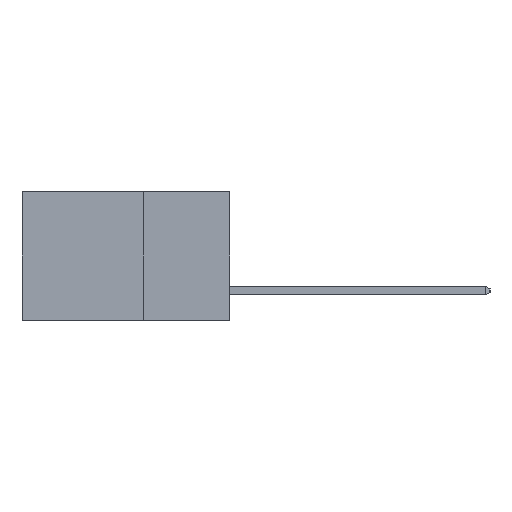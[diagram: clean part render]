
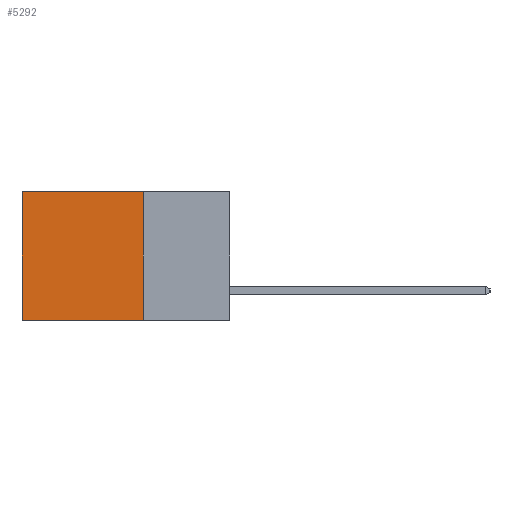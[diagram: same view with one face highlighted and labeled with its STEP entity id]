
A CAD part, left-side view. The second image highlights one B-rep face of the part: STEP entity #5292.
In plain terms, the highlighted planar face has unit normal (-1, 0, 0).
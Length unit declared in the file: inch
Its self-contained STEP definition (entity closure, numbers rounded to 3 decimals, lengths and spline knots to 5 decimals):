
#74 = VECTOR ( 'NONE', #10549, 39.37008 ) ;
#1083 = DIRECTION ( 'NONE',  ( 0., 0., -1. ) ) ;
#1556 = EDGE_CURVE ( 'NONE', #17391, #4035, #14110, .T. ) ;
#2933 = CARTESIAN_POINT ( 'NONE',  ( 0.298, 0.25, 0. ) ) ;
#3402 = VECTOR ( 'NONE', #12834, 39.37008 ) ;
#4035 = VERTEX_POINT ( 'NONE', #4414 ) ;
#4414 = CARTESIAN_POINT ( 'NONE',  ( 0.298, 0.6, -0.37 ) ) ;
#4563 = AXIS2_PLACEMENT_3D ( 'NONE', #9287, #10933, #1083 ) ;
#4794 = VECTOR ( 'NONE', #13952, 39.37008 ) ;
#5292 = ADVANCED_FACE ( 'NONE', ( #11680 ), #19150, .F. ) ;
#5662 = CARTESIAN_POINT ( 'NONE',  ( 0.298, 0.6, 0. ) ) ;
#5738 = CARTESIAN_POINT ( 'NONE',  ( 0.298, 0.6, 0. ) ) ;
#7088 = CARTESIAN_POINT ( 'NONE',  ( 0.298, 0.25, -0.37 ) ) ;
#7168 = DIRECTION ( 'NONE',  ( 0., 1., 0. ) ) ;
#7608 = LINE ( 'NONE', #7088, #11459 ) ;
#8453 = EDGE_CURVE ( 'NONE', #18607, #17391, #15561, .T. ) ;
#8903 = CARTESIAN_POINT ( 'NONE',  ( 0.298, 0.25, 0. ) ) ;
#9132 = CARTESIAN_POINT ( 'NONE',  ( 0.298, 0.25, -0.37 ) ) ;
#9287 = CARTESIAN_POINT ( 'NONE',  ( 0.298, 0.25, 0. ) ) ;
#9345 = ORIENTED_EDGE ( 'NONE', *, *, #14228, .F. ) ;
#10002 = CARTESIAN_POINT ( 'NONE',  ( 0.298, 0.25, 0. ) ) ;
#10549 = DIRECTION ( 'NONE',  ( 0., 0., -1. ) ) ;
#10933 = DIRECTION ( 'NONE',  ( 1., 0., 0. ) ) ;
#11366 = VERTEX_POINT ( 'NONE', #9132 ) ;
#11459 = VECTOR ( 'NONE', #7168, 39.37008 ) ;
#11680 = FACE_OUTER_BOUND ( 'NONE', #13837, .T. ) ;
#12834 = DIRECTION ( 'NONE',  ( 0., 1., 0. ) ) ;
#13837 = EDGE_LOOP ( 'NONE', ( #19566, #20930, #9345, #17321 ) ) ;
#13952 = DIRECTION ( 'NONE',  ( 0., 0., -1. ) ) ;
#14110 = LINE ( 'NONE', #5662, #4794 ) ;
#14228 = EDGE_CURVE ( 'NONE', #18607, #11366, #17602, .T. ) ;
#15561 = LINE ( 'NONE', #2933, #3402 ) ;
#16055 = EDGE_CURVE ( 'NONE', #11366, #4035, #7608, .T. ) ;
#17321 = ORIENTED_EDGE ( 'NONE', *, *, #8453, .T. ) ;
#17391 = VERTEX_POINT ( 'NONE', #5738 ) ;
#17602 = LINE ( 'NONE', #8903, #74 ) ;
#18607 = VERTEX_POINT ( 'NONE', #10002 ) ;
#19150 = PLANE ( 'NONE',  #4563 ) ;
#19566 = ORIENTED_EDGE ( 'NONE', *, *, #1556, .T. ) ;
#20930 = ORIENTED_EDGE ( 'NONE', *, *, #16055, .F. ) ;
